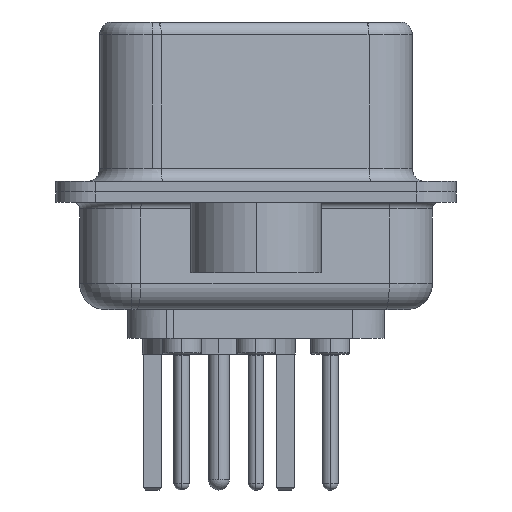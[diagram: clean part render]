
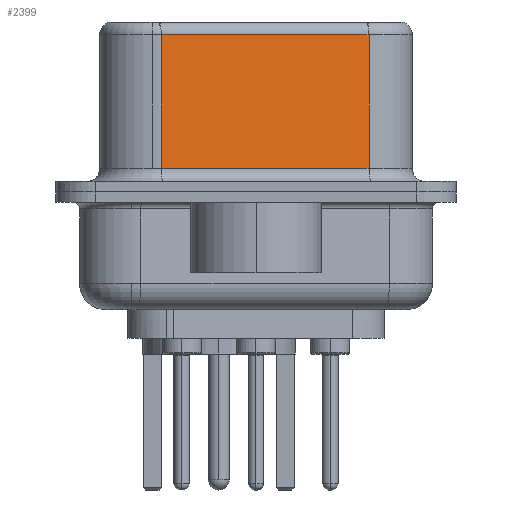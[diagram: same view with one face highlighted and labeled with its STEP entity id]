
A CAD part, left-side view. The second image highlights one B-rep face of the part: STEP entity #2399.
In plain terms, the highlighted planar face has unit normal (-0.985, -0.174, 0).
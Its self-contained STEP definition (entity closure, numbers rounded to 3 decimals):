
#241 = DIRECTION ( 'NONE',  ( 0.174, -0.985, 0. ) ) ;
#419 = CARTESIAN_POINT ( 'NONE',  ( 3.73, 3.628, 6.02 ) ) ;
#943 = FACE_OUTER_BOUND ( 'NONE', #15243, .T. ) ;
#2399 = ADVANCED_FACE ( 'NONE', ( #943 ), #5608, .F. ) ;
#4008 = VERTEX_POINT ( 'NONE', #25591 ) ;
#5608 = PLANE ( 'NONE',  #13076 ) ;
#6131 = VECTOR ( 'NONE', #32244, 1000. ) ;
#6503 = VECTOR ( 'NONE', #241, 1000. ) ;
#8242 = EDGE_CURVE ( 'NONE', #10808, #4008, #25117, .T. ) ;
#8421 = LINE ( 'NONE', #25128, #6503 ) ;
#10808 = VERTEX_POINT ( 'NONE', #419 ) ;
#11837 = CARTESIAN_POINT ( 'NONE',  ( 5.132, -4.322, 0.9 ) ) ;
#12102 = ORIENTED_EDGE ( 'NONE', *, *, #21646, .F. ) ;
#12782 = CARTESIAN_POINT ( 'NONE',  ( 5.132, -4.322, 6.52 ) ) ;
#13076 = AXIS2_PLACEMENT_3D ( 'NONE', #12782, #20674, #15652 ) ;
#13402 = EDGE_CURVE ( 'NONE', #28057, #10808, #21342, .T. ) ;
#13721 = EDGE_CURVE ( 'NONE', #4008, #18259, #8421, .T. ) ;
#14098 = CARTESIAN_POINT ( 'NONE',  ( 5.132, -4.322, 6.02 ) ) ;
#14181 = ORIENTED_EDGE ( 'NONE', *, *, #8242, .T. ) ;
#15036 = CARTESIAN_POINT ( 'NONE',  ( 3.73, 3.628, 6.52 ) ) ;
#15243 = EDGE_LOOP ( 'NONE', ( #12102, #30057, #14181, #17957 ) ) ;
#15652 = DIRECTION ( 'NONE',  ( -0.174, 0.985, 0. ) ) ;
#17422 = CARTESIAN_POINT ( 'NONE',  ( 5.132, -4.322, 6.52 ) ) ;
#17875 = DIRECTION ( 'NONE',  ( 0., 0., -1. ) ) ;
#17957 = ORIENTED_EDGE ( 'NONE', *, *, #13721, .T. ) ;
#18259 = VERTEX_POINT ( 'NONE', #11837 ) ;
#19934 = DIRECTION ( 'NONE',  ( 0., 0., -1. ) ) ;
#20674 = DIRECTION ( 'NONE',  ( 0.985, 0.174, 0. ) ) ;
#21342 = LINE ( 'NONE', #14098, #6131 ) ;
#21646 = EDGE_CURVE ( 'NONE', #28057, #18259, #26809, .T. ) ;
#22529 = VECTOR ( 'NONE', #19934, 1000. ) ;
#23104 = CARTESIAN_POINT ( 'NONE',  ( 5.132, -4.322, 6.02 ) ) ;
#25117 = LINE ( 'NONE', #15036, #32173 ) ;
#25128 = CARTESIAN_POINT ( 'NONE',  ( 5.132, -4.322, 0.9 ) ) ;
#25591 = CARTESIAN_POINT ( 'NONE',  ( 3.73, 3.628, 0.9 ) ) ;
#26809 = LINE ( 'NONE', #17422, #22529 ) ;
#28057 = VERTEX_POINT ( 'NONE', #23104 ) ;
#30057 = ORIENTED_EDGE ( 'NONE', *, *, #13402, .T. ) ;
#32173 = VECTOR ( 'NONE', #17875, 1000. ) ;
#32244 = DIRECTION ( 'NONE',  ( -0.174, 0.985, 0. ) ) ;
